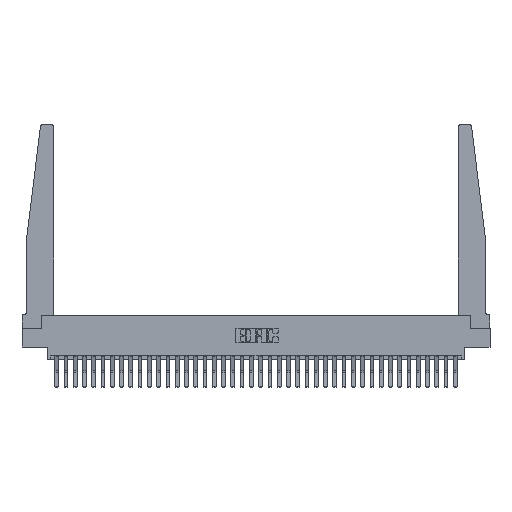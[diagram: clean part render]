
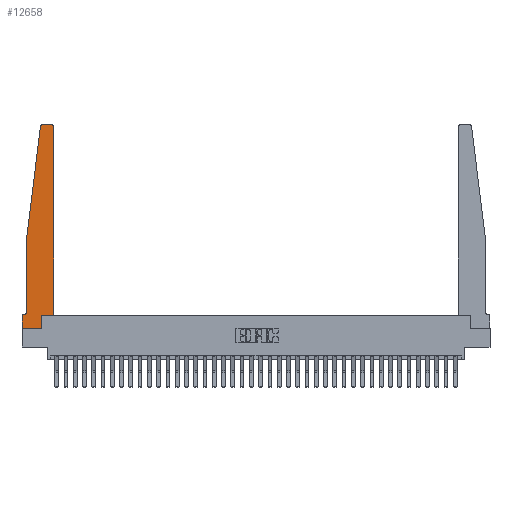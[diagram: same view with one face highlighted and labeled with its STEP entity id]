
A CAD part, top view. The second image highlights one B-rep face of the part: STEP entity #12658.
In plain terms, the highlighted planar face has unit normal (0, 0, 1).
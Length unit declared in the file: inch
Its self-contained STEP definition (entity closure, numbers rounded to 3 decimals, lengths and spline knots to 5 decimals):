
#119 = ORIENTED_EDGE ( 'NONE', *, *, #15003, .T. ) ;
#899 = EDGE_CURVE ( 'NONE', #22392, #32785, #24375, .T. ) ;
#1803 = CARTESIAN_POINT ( 'NONE',  ( 0.395, 2.72, 0.37 ) ) ;
#1977 = CARTESIAN_POINT ( 'NONE',  ( 0.2605, 0.18, 0.37 ) ) ;
#2531 = AXIS2_PLACEMENT_3D ( 'NONE', #1803, #19937, #4388 ) ;
#3097 = DIRECTION ( 'NONE',  ( 0., 0., 1. ) ) ;
#3847 = DIRECTION ( 'NONE',  ( 0., 1., 0. ) ) ;
#3864 = CARTESIAN_POINT ( 'NONE',  ( 0.065, 0.2375, 0.37 ) ) ;
#4126 = VERTEX_POINT ( 'NONE', #20677 ) ;
#4388 = DIRECTION ( 'NONE',  ( 1., 0., 0. ) ) ;
#4531 = ORIENTED_EDGE ( 'NONE', *, *, #22515, .T. ) ;
#5027 = VECTOR ( 'NONE', #28968, 39.37008 ) ;
#5059 = CARTESIAN_POINT ( 'NONE',  ( 0.065, 0.1875, 0.37 ) ) ;
#5703 = DIRECTION ( 'NONE',  ( 0., -1., 0. ) ) ;
#5733 = VERTEX_POINT ( 'NONE', #16204 ) ;
#6155 = ORIENTED_EDGE ( 'NONE', *, *, #14796, .T. ) ;
#7747 = VECTOR ( 'NONE', #14843, 39.37008 ) ;
#7887 = CARTESIAN_POINT ( 'NONE',  ( 0.2605, 0.18, 0.37 ) ) ;
#8145 = EDGE_LOOP ( 'NONE', ( #23651, #9874, #30362, #23999, #8614, #119, #15504, #23966, #21558, #19960, #4531, #6155 ) ) ;
#8198 = CARTESIAN_POINT ( 'NONE',  ( 0., 0.1875, 0.37 ) ) ;
#8614 = ORIENTED_EDGE ( 'NONE', *, *, #31880, .T. ) ;
#8949 = CARTESIAN_POINT ( 'NONE',  ( 0.2605, 0., 0.37 ) ) ;
#9682 = VERTEX_POINT ( 'NONE', #11876 ) ;
#9874 = ORIENTED_EDGE ( 'NONE', *, *, #23970, .T. ) ;
#10691 = EDGE_CURVE ( 'NONE', #17489, #27947, #15676, .T. ) ;
#11615 = VECTOR ( 'NONE', #31786, 39.37008 ) ;
#11876 = CARTESIAN_POINT ( 'NONE',  ( 0.24675, 2.72367, 0.37 ) ) ;
#12552 = LINE ( 'NONE', #5059, #18643 ) ;
#12658 = ADVANCED_FACE ( 'NONE', ( #14378 ), #31463, .T. ) ;
#12696 = EDGE_CURVE ( 'NONE', #4126, #17489, #13569, .T. ) ;
#12713 = EDGE_CURVE ( 'NONE', #9682, #22392, #19651, .T. ) ;
#12750 = VECTOR ( 'NONE', #5703, 39.37008 ) ;
#12899 = CIRCLE ( 'NONE', #16093, 0.05 ) ;
#13084 = CARTESIAN_POINT ( 'NONE',  ( 0., 0., 0.37 ) ) ;
#13123 = DIRECTION ( 'NONE',  ( 0., 0., -1. ) ) ;
#13301 = CARTESIAN_POINT ( 'NONE',  ( 0.015, 0.1875, 0.37 ) ) ;
#13569 = LINE ( 'NONE', #23790, #12750 ) ;
#13598 = VERTEX_POINT ( 'NONE', #1977 ) ;
#13824 = VERTEX_POINT ( 'NONE', #13301 ) ;
#13905 = CARTESIAN_POINT ( 'NONE',  ( 0.065, 1.25, 0.37 ) ) ;
#14176 = CARTESIAN_POINT ( 'NONE',  ( 0.425, 0.18, 0.37 ) ) ;
#14378 = FACE_OUTER_BOUND ( 'NONE', #8145, .T. ) ;
#14796 = EDGE_CURVE ( 'NONE', #15918, #15932, #18274, .T. ) ;
#14843 = DIRECTION ( 'NONE',  ( -1., 0., 0. ) ) ;
#15003 = EDGE_CURVE ( 'NONE', #13824, #4126, #12552, .T. ) ;
#15110 = DIRECTION ( 'NONE',  ( 0., 0., 1. ) ) ;
#15504 = ORIENTED_EDGE ( 'NONE', *, *, #12696, .T. ) ;
#15676 = LINE ( 'NONE', #13084, #28549 ) ;
#15690 = DIRECTION ( 'NONE',  ( 1., 0., 0. ) ) ;
#15918 = VERTEX_POINT ( 'NONE', #16354 ) ;
#15932 = VERTEX_POINT ( 'NONE', #21651 ) ;
#16093 = AXIS2_PLACEMENT_3D ( 'NONE', #28545, #13123, #31155 ) ;
#16204 = CARTESIAN_POINT ( 'NONE',  ( 0.27653, 2.75, 0.37 ) ) ;
#16354 = CARTESIAN_POINT ( 'NONE',  ( 0.425, 2.72, 0.37 ) ) ;
#17489 = VERTEX_POINT ( 'NONE', #17607 ) ;
#17607 = CARTESIAN_POINT ( 'NONE',  ( 0., 0., 0.37 ) ) ;
#17824 = CIRCLE ( 'NONE', #27364, 0.03 ) ;
#18184 = CARTESIAN_POINT ( 'NONE',  ( 0.425, 0.18, 0.37 ) ) ;
#18217 = VECTOR ( 'NONE', #31145, 39.37008 ) ;
#18274 = CIRCLE ( 'NONE', #2531, 0.03 ) ;
#18643 = VECTOR ( 'NONE', #33417, 39.37008 ) ;
#19007 = LINE ( 'NONE', #7887, #18217 ) ;
#19651 = LINE ( 'NONE', #29072, #5027 ) ;
#19937 = DIRECTION ( 'NONE',  ( 0., 0., 1. ) ) ;
#19960 = ORIENTED_EDGE ( 'NONE', *, *, #32660, .T. ) ;
#20152 = LINE ( 'NONE', #29173, #11615 ) ;
#20677 = CARTESIAN_POINT ( 'NONE',  ( 0., 0.1875, 0.37 ) ) ;
#20948 = AXIS2_PLACEMENT_3D ( 'NONE', #8198, #3097, #21223 ) ;
#21223 = DIRECTION ( 'NONE',  ( 1., 0., 0. ) ) ;
#21558 = ORIENTED_EDGE ( 'NONE', *, *, #23445, .T. ) ;
#21651 = CARTESIAN_POINT ( 'NONE',  ( 0.395, 2.75, 0.37 ) ) ;
#21922 = EDGE_CURVE ( 'NONE', #15932, #5733, #27528, .T. ) ;
#22328 = CARTESIAN_POINT ( 'NONE',  ( 0.065, 1.25, 0.37 ) ) ;
#22392 = VERTEX_POINT ( 'NONE', #13905 ) ;
#22515 = EDGE_CURVE ( 'NONE', #31248, #15918, #31953, .T. ) ;
#23445 = EDGE_CURVE ( 'NONE', #27947, #13598, #19007, .T. ) ;
#23651 = ORIENTED_EDGE ( 'NONE', *, *, #21922, .T. ) ;
#23790 = CARTESIAN_POINT ( 'NONE',  ( 0., 0., 0.37 ) ) ;
#23966 = ORIENTED_EDGE ( 'NONE', *, *, #10691, .T. ) ;
#23970 = EDGE_CURVE ( 'NONE', #5733, #9682, #17824, .T. ) ;
#23999 = ORIENTED_EDGE ( 'NONE', *, *, #899, .T. ) ;
#24375 = LINE ( 'NONE', #22328, #30402 ) ;
#25109 = VECTOR ( 'NONE', #3847, 39.37008 ) ;
#27364 = AXIS2_PLACEMENT_3D ( 'NONE', #30543, #15110, #33147 ) ;
#27528 = LINE ( 'NONE', #30263, #7747 ) ;
#27947 = VERTEX_POINT ( 'NONE', #8949 ) ;
#28545 = CARTESIAN_POINT ( 'NONE',  ( 0.015, 0.2375, 0.37 ) ) ;
#28549 = VECTOR ( 'NONE', #15690, 39.37008 ) ;
#28968 = DIRECTION ( 'NONE',  ( -0.122, -0.992, 0. ) ) ;
#29072 = CARTESIAN_POINT ( 'NONE',  ( 0.065, 1.25, 0.37 ) ) ;
#29173 = CARTESIAN_POINT ( 'NONE',  ( 0.425, 0.18, 0.37 ) ) ;
#30263 = CARTESIAN_POINT ( 'NONE',  ( 0.25, 2.75, 0.37 ) ) ;
#30362 = ORIENTED_EDGE ( 'NONE', *, *, #12713, .T. ) ;
#30402 = VECTOR ( 'NONE', #32569, 39.37008 ) ;
#30543 = CARTESIAN_POINT ( 'NONE',  ( 0.27653, 2.72, 0.37 ) ) ;
#31145 = DIRECTION ( 'NONE',  ( 0., 1., 0. ) ) ;
#31155 = DIRECTION ( 'NONE',  ( -1., 0., 0. ) ) ;
#31248 = VERTEX_POINT ( 'NONE', #18184 ) ;
#31463 = PLANE ( 'NONE',  #20948 ) ;
#31786 = DIRECTION ( 'NONE',  ( 1., 0., 0. ) ) ;
#31880 = EDGE_CURVE ( 'NONE', #32785, #13824, #12899, .T. ) ;
#31953 = LINE ( 'NONE', #14176, #25109 ) ;
#32569 = DIRECTION ( 'NONE',  ( 0., -1., 0. ) ) ;
#32660 = EDGE_CURVE ( 'NONE', #13598, #31248, #20152, .T. ) ;
#32785 = VERTEX_POINT ( 'NONE', #3864 ) ;
#33147 = DIRECTION ( 'NONE',  ( 1., 0., 0. ) ) ;
#33417 = DIRECTION ( 'NONE',  ( -1., 0., 0. ) ) ;
